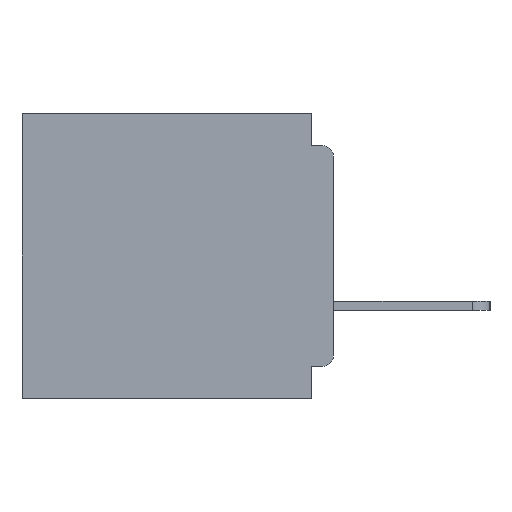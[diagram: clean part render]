
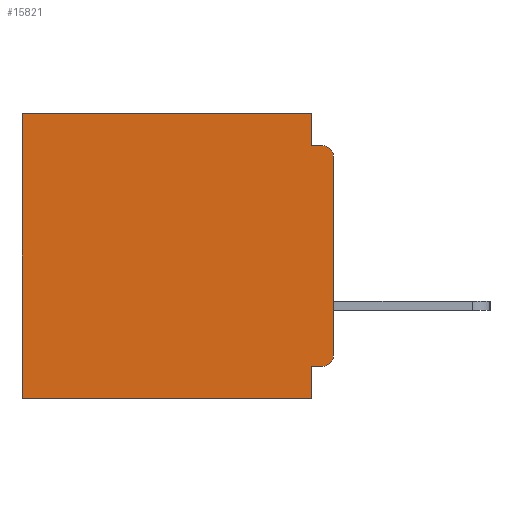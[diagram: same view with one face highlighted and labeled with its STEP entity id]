
A CAD part, left-side view. The second image highlights one B-rep face of the part: STEP entity #15821.
In plain terms, the highlighted planar face has unit normal (-1, 0, 0).
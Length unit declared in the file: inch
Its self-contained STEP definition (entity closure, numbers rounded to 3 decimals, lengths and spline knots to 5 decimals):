
#257 = EDGE_CURVE ( 'NONE', #28124, #3002, #8243, .T. ) ;
#315 = EDGE_LOOP ( 'NONE', ( #24612, #25145, #31542, #32880, #15361, #21224, #9657, #30892, #4036, #9029 ) ) ;
#855 = EDGE_CURVE ( 'NONE', #21932, #4270, #3102, .T. ) ;
#1403 = CARTESIAN_POINT ( 'NONE',  ( 0.3, 0., -0.4 ) ) ;
#1522 = DIRECTION ( 'NONE',  ( 1., 0., 0. ) ) ;
#1659 = CARTESIAN_POINT ( 'NONE',  ( 0.3, 0., -0.355 ) ) ;
#1815 = AXIS2_PLACEMENT_3D ( 'NONE', #33854, #26817, #31050 ) ;
#1828 = CARTESIAN_POINT ( 'NONE',  ( 0.3, 0.031, -0.4 ) ) ;
#1992 = DIRECTION ( 'NONE',  ( 0., 1., 0. ) ) ;
#2091 = CARTESIAN_POINT ( 'NONE',  ( 0.3, 0., 0. ) ) ;
#2143 = VECTOR ( 'NONE', #9264, 39.37008 ) ;
#2280 = LINE ( 'NONE', #1659, #16674 ) ;
#2970 = EDGE_CURVE ( 'NONE', #5952, #4270, #12324, .T. ) ;
#3002 = VERTEX_POINT ( 'NONE', #10598 ) ;
#3102 = LINE ( 'NONE', #11874, #15828 ) ;
#3155 = DIRECTION ( 'NONE',  ( 0., 1., 0. ) ) ;
#3553 = LINE ( 'NONE', #16007, #31148 ) ;
#4036 = ORIENTED_EDGE ( 'NONE', *, *, #8341, .F. ) ;
#4206 = VERTEX_POINT ( 'NONE', #14960 ) ;
#4258 = CARTESIAN_POINT ( 'NONE',  ( 0.3, 0.031, 0. ) ) ;
#4270 = VERTEX_POINT ( 'NONE', #5873 ) ;
#5873 = CARTESIAN_POINT ( 'NONE',  ( 0.3, 0.437, -0.4 ) ) ;
#5952 = VERTEX_POINT ( 'NONE', #17702 ) ;
#7451 = LINE ( 'NONE', #2091, #21734 ) ;
#8243 = CIRCLE ( 'NONE', #1815, 0.015 ) ;
#8341 = EDGE_CURVE ( 'NONE', #34470, #4206, #2280, .T. ) ;
#9029 = ORIENTED_EDGE ( 'NONE', *, *, #15580, .T. ) ;
#9264 = DIRECTION ( 'NONE',  ( 0., 0., -1. ) ) ;
#9657 = ORIENTED_EDGE ( 'NONE', *, *, #855, .F. ) ;
#10598 = CARTESIAN_POINT ( 'NONE',  ( 0.3, 0.015, -0.045 ) ) ;
#11269 = CARTESIAN_POINT ( 'NONE',  ( 0.3, 0.015, -0.34 ) ) ;
#11281 = CARTESIAN_POINT ( 'NONE',  ( 0.3, 0., -0.045 ) ) ;
#11874 = CARTESIAN_POINT ( 'NONE',  ( 0.3, 0., -0.4 ) ) ;
#12324 = LINE ( 'NONE', #28377, #25688 ) ;
#12653 = FACE_OUTER_BOUND ( 'NONE', #315, .T. ) ;
#12984 = EDGE_CURVE ( 'NONE', #17970, #25057, #3553, .T. ) ;
#14025 = DIRECTION ( 'NONE',  ( 0., 0., -1. ) ) ;
#14123 = LINE ( 'NONE', #1828, #34312 ) ;
#14635 = EDGE_CURVE ( 'NONE', #28124, #23666, #16533, .T. ) ;
#14655 = CARTESIAN_POINT ( 'NONE',  ( 0.3, 0.015, -0.355 ) ) ;
#14960 = CARTESIAN_POINT ( 'NONE',  ( 0.3, 0.031, -0.355 ) ) ;
#15336 = DIRECTION ( 'NONE',  ( 0., 0., -1. ) ) ;
#15361 = ORIENTED_EDGE ( 'NONE', *, *, #23845, .T. ) ;
#15580 = EDGE_CURVE ( 'NONE', #34470, #23666, #33375, .T. ) ;
#15821 = ADVANCED_FACE ( 'NONE', ( #12653 ), #17724, .F. ) ;
#15828 = VECTOR ( 'NONE', #3155, 39.37008 ) ;
#15875 = VECTOR ( 'NONE', #29910, 39.37008 ) ;
#16007 = CARTESIAN_POINT ( 'NONE',  ( 0.3, 0.031, 0. ) ) ;
#16533 = LINE ( 'NONE', #30585, #2143 ) ;
#16674 = VECTOR ( 'NONE', #1992, 39.37008 ) ;
#17702 = CARTESIAN_POINT ( 'NONE',  ( 0.3, 0.437, 0. ) ) ;
#17724 = PLANE ( 'NONE',  #27886 ) ;
#17970 = VERTEX_POINT ( 'NONE', #4258 ) ;
#20426 = DIRECTION ( 'NONE',  ( 0., 0., -1. ) ) ;
#20951 = DIRECTION ( 'NONE',  ( 0., 1., 0. ) ) ;
#21224 = ORIENTED_EDGE ( 'NONE', *, *, #2970, .T. ) ;
#21734 = VECTOR ( 'NONE', #20951, 39.37008 ) ;
#21932 = VERTEX_POINT ( 'NONE', #24136 ) ;
#23554 = CARTESIAN_POINT ( 'NONE',  ( 0.3, 0.031, -0.045 ) ) ;
#23666 = VERTEX_POINT ( 'NONE', #25362 ) ;
#23845 = EDGE_CURVE ( 'NONE', #17970, #5952, #7451, .T. ) ;
#24136 = CARTESIAN_POINT ( 'NONE',  ( 0.3, 0.031, -0.4 ) ) ;
#24612 = ORIENTED_EDGE ( 'NONE', *, *, #14635, .F. ) ;
#25057 = VERTEX_POINT ( 'NONE', #23554 ) ;
#25145 = ORIENTED_EDGE ( 'NONE', *, *, #257, .T. ) ;
#25362 = CARTESIAN_POINT ( 'NONE',  ( 0.3, 0., -0.34 ) ) ;
#25688 = VECTOR ( 'NONE', #26737, 39.37008 ) ;
#26737 = DIRECTION ( 'NONE',  ( 0., 0., -1. ) ) ;
#26778 = AXIS2_PLACEMENT_3D ( 'NONE', #11269, #29899, #14025 ) ;
#26817 = DIRECTION ( 'NONE',  ( -1., 0., 0. ) ) ;
#27522 = CARTESIAN_POINT ( 'NONE',  ( 0.3, 0., -0.06 ) ) ;
#27886 = AXIS2_PLACEMENT_3D ( 'NONE', #1403, #1522, #20426 ) ;
#28124 = VERTEX_POINT ( 'NONE', #27522 ) ;
#28377 = CARTESIAN_POINT ( 'NONE',  ( 0.3, 0.437, -0.4 ) ) ;
#28383 = EDGE_CURVE ( 'NONE', #4206, #21932, #14123, .T. ) ;
#29133 = LINE ( 'NONE', #11281, #15875 ) ;
#29899 = DIRECTION ( 'NONE',  ( -1., 0., 0. ) ) ;
#29910 = DIRECTION ( 'NONE',  ( 0., -1., 0. ) ) ;
#30585 = CARTESIAN_POINT ( 'NONE',  ( 0.3, 0., -0.4 ) ) ;
#30892 = ORIENTED_EDGE ( 'NONE', *, *, #28383, .F. ) ;
#31050 = DIRECTION ( 'NONE',  ( 0., 0., -1. ) ) ;
#31148 = VECTOR ( 'NONE', #34409, 39.37008 ) ;
#31542 = ORIENTED_EDGE ( 'NONE', *, *, #33296, .F. ) ;
#32880 = ORIENTED_EDGE ( 'NONE', *, *, #12984, .F. ) ;
#33296 = EDGE_CURVE ( 'NONE', #25057, #3002, #29133, .T. ) ;
#33375 = CIRCLE ( 'NONE', #26778, 0.015 ) ;
#33854 = CARTESIAN_POINT ( 'NONE',  ( 0.3, 0.015, -0.06 ) ) ;
#34312 = VECTOR ( 'NONE', #15336, 39.37008 ) ;
#34409 = DIRECTION ( 'NONE',  ( 0., 0., -1. ) ) ;
#34470 = VERTEX_POINT ( 'NONE', #14655 ) ;
